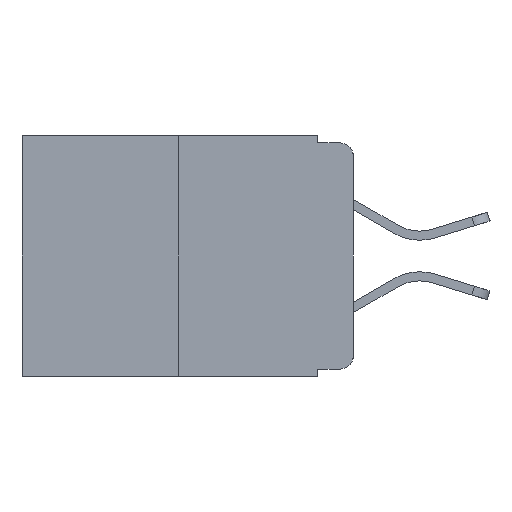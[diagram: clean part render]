
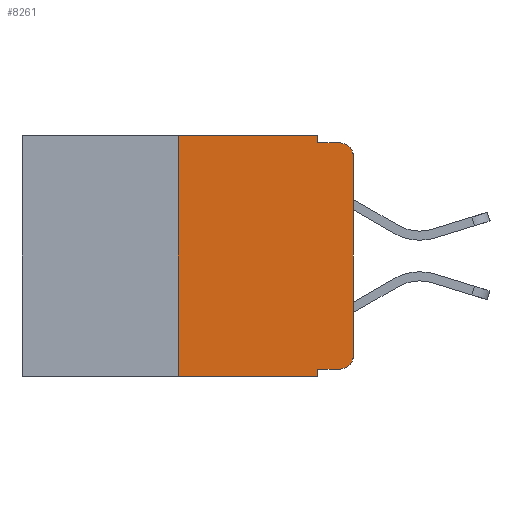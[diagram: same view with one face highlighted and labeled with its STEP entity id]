
A CAD part, left-side view. The second image highlights one B-rep face of the part: STEP entity #8261.
In plain terms, the highlighted planar face has unit normal (-1, 0, 0).
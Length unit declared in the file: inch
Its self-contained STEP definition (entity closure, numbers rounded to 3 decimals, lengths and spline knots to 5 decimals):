
#11 = ORIENTED_EDGE ( 'NONE', *, *, #2609, .F. ) ;
#161 = ORIENTED_EDGE ( 'NONE', *, *, #5216, .T. ) ;
#469 = VERTEX_POINT ( 'NONE', #9804 ) ;
#487 = ORIENTED_EDGE ( 'NONE', *, *, #4713, .F. ) ;
#557 = VERTEX_POINT ( 'NONE', #10182 ) ;
#633 = VERTEX_POINT ( 'NONE', #2640 ) ;
#682 = CARTESIAN_POINT ( 'NONE',  ( 0., 0.051, -0.343 ) ) ;
#869 = LINE ( 'NONE', #8000, #5019 ) ;
#1016 = DIRECTION ( 'NONE',  ( 0., -1., 0. ) ) ;
#1057 = CARTESIAN_POINT ( 'NONE',  ( 0., 0.051, 0. ) ) ;
#1207 = CARTESIAN_POINT ( 'NONE',  ( 0., 0.473, 0. ) ) ;
#1238 = VERTEX_POINT ( 'NONE', #7995 ) ;
#1633 = LINE ( 'NONE', #4555, #5635 ) ;
#1839 = VERTEX_POINT ( 'NONE', #8402 ) ;
#1863 = EDGE_CURVE ( 'NONE', #1839, #9822, #5076, .T. ) ;
#2255 = DIRECTION ( 'NONE',  ( 0., -1., 0. ) ) ;
#2463 = CIRCLE ( 'NONE', #5952, 0.02 ) ;
#2609 = EDGE_CURVE ( 'NONE', #9154, #6695, #1633, .T. ) ;
#2640 = CARTESIAN_POINT ( 'NONE',  ( 0., 0.051, 0. ) ) ;
#2705 = LINE ( 'NONE', #7792, #4541 ) ;
#2715 = LINE ( 'NONE', #1057, #6519 ) ;
#2949 = CIRCLE ( 'NONE', #5072, 0.02 ) ;
#3012 = EDGE_CURVE ( 'NONE', #1839, #4610, #7378, .T. ) ;
#3022 = VECTOR ( 'NONE', #7982, 39.37008 ) ;
#3208 = CARTESIAN_POINT ( 'NONE',  ( 0., 0.02, -0.313 ) ) ;
#3440 = ORIENTED_EDGE ( 'NONE', *, *, #4213, .F. ) ;
#3486 = VECTOR ( 'NONE', #2255, 39.37008 ) ;
#3504 = DIRECTION ( 'NONE',  ( -1., 0., 0. ) ) ;
#3570 = EDGE_CURVE ( 'NONE', #6695, #633, #5730, .T. ) ;
#3635 = CARTESIAN_POINT ( 'NONE',  ( 0., 0.02, -0.333 ) ) ;
#3690 = CARTESIAN_POINT ( 'NONE',  ( 0., 0., 0. ) ) ;
#3860 = DIRECTION ( 'NONE',  ( 1., 0., 0. ) ) ;
#3932 = ORIENTED_EDGE ( 'NONE', *, *, #3570, .F. ) ;
#4008 = DIRECTION ( 'NONE',  ( 0., 0., -1. ) ) ;
#4148 = EDGE_CURVE ( 'NONE', #9154, #4610, #869, .T. ) ;
#4213 = EDGE_CURVE ( 'NONE', #633, #557, #2715, .T. ) ;
#4336 = FACE_OUTER_BOUND ( 'NONE', #6330, .T. ) ;
#4541 = VECTOR ( 'NONE', #8473, 39.37008 ) ;
#4555 = CARTESIAN_POINT ( 'NONE',  ( 0., 0.25, 0. ) ) ;
#4610 = VERTEX_POINT ( 'NONE', #682 ) ;
#4648 = VECTOR ( 'NONE', #8954, 39.37008 ) ;
#4713 = EDGE_CURVE ( 'NONE', #557, #469, #2705, .T. ) ;
#5019 = VECTOR ( 'NONE', #1016, 39.37008 ) ;
#5072 = AXIS2_PLACEMENT_3D ( 'NONE', #8014, #3504, #8769 ) ;
#5076 = LINE ( 'NONE', #8009, #3022 ) ;
#5216 = EDGE_CURVE ( 'NONE', #7662, #469, #2949, .T. ) ;
#5635 = VECTOR ( 'NONE', #7599, 39.37008 ) ;
#5730 = LINE ( 'NONE', #1207, #3486 ) ;
#5952 = AXIS2_PLACEMENT_3D ( 'NONE', #3208, #8504, #4008 ) ;
#5960 = PLANE ( 'NONE',  #8791 ) ;
#6108 = CARTESIAN_POINT ( 'NONE',  ( 0., 0., -0.03 ) ) ;
#6206 = EDGE_CURVE ( 'NONE', #1238, #7662, #6380, .T. ) ;
#6330 = EDGE_LOOP ( 'NONE', ( #7799, #161, #487, #3440, #3932, #11, #8862, #9319, #9792, #8286 ) ) ;
#6380 = LINE ( 'NONE', #3690, #4648 ) ;
#6519 = VECTOR ( 'NONE', #8379, 39.37008 ) ;
#6558 = CARTESIAN_POINT ( 'NONE',  ( 0., 0.25, -0.343 ) ) ;
#6695 = VERTEX_POINT ( 'NONE', #8745 ) ;
#7126 = CARTESIAN_POINT ( 'NONE',  ( 0., 0.051, 0. ) ) ;
#7135 = DIRECTION ( 'NONE',  ( 0., 0., -1. ) ) ;
#7145 = VECTOR ( 'NONE', #7135, 39.37008 ) ;
#7378 = LINE ( 'NONE', #7126, #7145 ) ;
#7599 = DIRECTION ( 'NONE',  ( 0., 0., 1. ) ) ;
#7662 = VERTEX_POINT ( 'NONE', #6108 ) ;
#7780 = EDGE_CURVE ( 'NONE', #9822, #1238, #2463, .T. ) ;
#7792 = CARTESIAN_POINT ( 'NONE',  ( 0., 0.051, -0.01 ) ) ;
#7799 = ORIENTED_EDGE ( 'NONE', *, *, #6206, .T. ) ;
#7982 = DIRECTION ( 'NONE',  ( 0., -1., 0. ) ) ;
#7995 = CARTESIAN_POINT ( 'NONE',  ( 0., 0., -0.313 ) ) ;
#8000 = CARTESIAN_POINT ( 'NONE',  ( 0., 0.473, -0.343 ) ) ;
#8009 = CARTESIAN_POINT ( 'NONE',  ( 0., 0.051, -0.333 ) ) ;
#8014 = CARTESIAN_POINT ( 'NONE',  ( 0., 0.02, -0.03 ) ) ;
#8261 = ADVANCED_FACE ( 'NONE', ( #4336 ), #5960, .F. ) ;
#8286 = ORIENTED_EDGE ( 'NONE', *, *, #7780, .T. ) ;
#8376 = CARTESIAN_POINT ( 'NONE',  ( 0., 0.473, 0. ) ) ;
#8379 = DIRECTION ( 'NONE',  ( 0., 0., -1. ) ) ;
#8402 = CARTESIAN_POINT ( 'NONE',  ( 0., 0.051, -0.333 ) ) ;
#8473 = DIRECTION ( 'NONE',  ( 0., -1., 0. ) ) ;
#8504 = DIRECTION ( 'NONE',  ( -1., 0., 0. ) ) ;
#8745 = CARTESIAN_POINT ( 'NONE',  ( 0., 0.25, 0. ) ) ;
#8769 = DIRECTION ( 'NONE',  ( 0., 0., -1. ) ) ;
#8791 = AXIS2_PLACEMENT_3D ( 'NONE', #8376, #3860, #9112 ) ;
#8862 = ORIENTED_EDGE ( 'NONE', *, *, #4148, .T. ) ;
#8954 = DIRECTION ( 'NONE',  ( 0., 0., 1. ) ) ;
#9112 = DIRECTION ( 'NONE',  ( 0., 0., -1. ) ) ;
#9154 = VERTEX_POINT ( 'NONE', #6558 ) ;
#9319 = ORIENTED_EDGE ( 'NONE', *, *, #3012, .F. ) ;
#9792 = ORIENTED_EDGE ( 'NONE', *, *, #1863, .T. ) ;
#9804 = CARTESIAN_POINT ( 'NONE',  ( 0., 0.02, -0.01 ) ) ;
#9822 = VERTEX_POINT ( 'NONE', #3635 ) ;
#10182 = CARTESIAN_POINT ( 'NONE',  ( 0., 0.051, -0.01 ) ) ;
